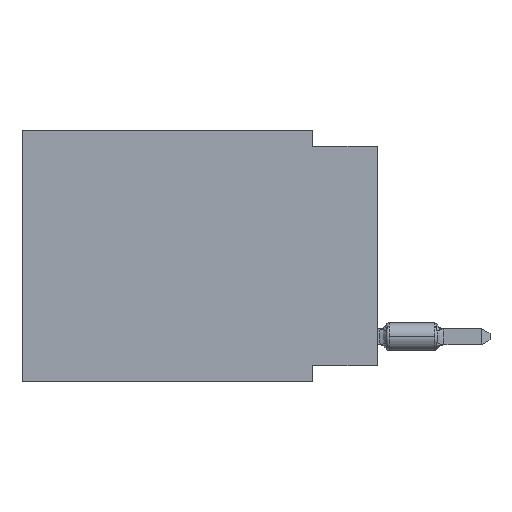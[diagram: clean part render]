
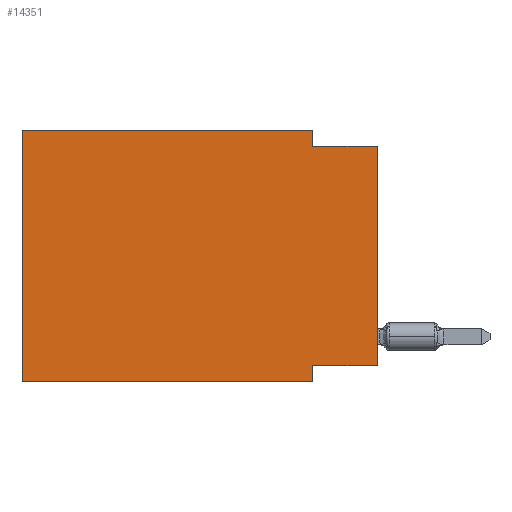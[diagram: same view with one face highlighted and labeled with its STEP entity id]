
A CAD part, left-side view. The second image highlights one B-rep face of the part: STEP entity #14351.
In plain terms, the highlighted planar face has unit normal (-1, 0, 0).
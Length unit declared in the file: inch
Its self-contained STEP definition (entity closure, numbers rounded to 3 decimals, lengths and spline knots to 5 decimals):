
#450 = DIRECTION ( 'NONE',  ( 0., 0., -1. ) ) ;
#493 = CARTESIAN_POINT ( 'NONE',  ( 0., 0.1, -0.39 ) ) ;
#547 = EDGE_CURVE ( 'NONE', #9017, #11128, #4218, .T. ) ;
#748 = DIRECTION ( 'NONE',  ( 0., 0., -1. ) ) ;
#989 = CARTESIAN_POINT ( 'NONE',  ( 0., 0.1, -0.365 ) ) ;
#1111 = CARTESIAN_POINT ( 'NONE',  ( 0., 0., -0.365 ) ) ;
#1274 = DIRECTION ( 'NONE',  ( 0., 0., -1. ) ) ;
#1516 = EDGE_CURVE ( 'NONE', #4479, #1922, #7244, .T. ) ;
#1914 = EDGE_CURVE ( 'NONE', #4148, #11128, #11303, .T. ) ;
#1922 = VERTEX_POINT ( 'NONE', #7546 ) ;
#2011 = ORIENTED_EDGE ( 'NONE', *, *, #15086, .T. ) ;
#2203 = CARTESIAN_POINT ( 'NONE',  ( 0., 0., -0.025 ) ) ;
#2472 = DIRECTION ( 'NONE',  ( 0., 1., 0. ) ) ;
#2761 = ORIENTED_EDGE ( 'NONE', *, *, #13108, .F. ) ;
#2795 = CARTESIAN_POINT ( 'NONE',  ( 0., 0., -0.365 ) ) ;
#2807 = CARTESIAN_POINT ( 'NONE',  ( 0., 0.1, 0. ) ) ;
#3110 = CARTESIAN_POINT ( 'NONE',  ( 0., 0.55, -0.39 ) ) ;
#3275 = LINE ( 'NONE', #16688, #9302 ) ;
#3716 = LINE ( 'NONE', #4912, #11057 ) ;
#4130 = VECTOR ( 'NONE', #748, 39.37008 ) ;
#4148 = VERTEX_POINT ( 'NONE', #2795 ) ;
#4209 = CARTESIAN_POINT ( 'NONE',  ( 0., 0.1, 0. ) ) ;
#4218 = LINE ( 'NONE', #9438, #11420 ) ;
#4401 = CARTESIAN_POINT ( 'NONE',  ( 0., 0.1, -0.025 ) ) ;
#4479 = VERTEX_POINT ( 'NONE', #989 ) ;
#4912 = CARTESIAN_POINT ( 'NONE',  ( 0., 0.55, -0.39 ) ) ;
#5392 = AXIS2_PLACEMENT_3D ( 'NONE', #11534, #10338, #1274 ) ;
#6012 = CARTESIAN_POINT ( 'NONE',  ( 0., 0., 0. ) ) ;
#6150 = ORIENTED_EDGE ( 'NONE', *, *, #10513, .F. ) ;
#6856 = DIRECTION ( 'NONE',  ( 0., -1., 0. ) ) ;
#7154 = EDGE_CURVE ( 'NONE', #13836, #11125, #3275, .T. ) ;
#7244 = LINE ( 'NONE', #493, #4130 ) ;
#7546 = CARTESIAN_POINT ( 'NONE',  ( 0., 0.1, -0.39 ) ) ;
#8159 = DIRECTION ( 'NONE',  ( 0., -1., 0. ) ) ;
#8424 = VECTOR ( 'NONE', #450, 39.37008 ) ;
#8580 = DIRECTION ( 'NONE',  ( 0., 0., 1. ) ) ;
#8835 = EDGE_LOOP ( 'NONE', ( #12155, #10376, #6150, #11674, #10535, #2011, #12660, #2761 ) ) ;
#9017 = VERTEX_POINT ( 'NONE', #4401 ) ;
#9302 = VECTOR ( 'NONE', #8580, 39.37008 ) ;
#9438 = CARTESIAN_POINT ( 'NONE',  ( 0., 0., -0.025 ) ) ;
#9688 = VERTEX_POINT ( 'NONE', #2807 ) ;
#10018 = VECTOR ( 'NONE', #2472, 39.37008 ) ;
#10338 = DIRECTION ( 'NONE',  ( 1., 0., 0. ) ) ;
#10376 = ORIENTED_EDGE ( 'NONE', *, *, #547, .F. ) ;
#10513 = EDGE_CURVE ( 'NONE', #9688, #9017, #13530, .T. ) ;
#10535 = ORIENTED_EDGE ( 'NONE', *, *, #7154, .F. ) ;
#10608 = LINE ( 'NONE', #13252, #14304 ) ;
#11057 = VECTOR ( 'NONE', #16623, 39.37008 ) ;
#11125 = VERTEX_POINT ( 'NONE', #11599 ) ;
#11128 = VERTEX_POINT ( 'NONE', #2203 ) ;
#11303 = LINE ( 'NONE', #6012, #16416 ) ;
#11420 = VECTOR ( 'NONE', #8159, 39.37008 ) ;
#11534 = CARTESIAN_POINT ( 'NONE',  ( 0., 0.55, 0. ) ) ;
#11599 = CARTESIAN_POINT ( 'NONE',  ( 0., 0.55, 0. ) ) ;
#11674 = ORIENTED_EDGE ( 'NONE', *, *, #15645, .F. ) ;
#12155 = ORIENTED_EDGE ( 'NONE', *, *, #1914, .T. ) ;
#12660 = ORIENTED_EDGE ( 'NONE', *, *, #1516, .F. ) ;
#12980 = PLANE ( 'NONE',  #5392 ) ;
#13108 = EDGE_CURVE ( 'NONE', #4148, #4479, #16830, .T. ) ;
#13252 = CARTESIAN_POINT ( 'NONE',  ( 0., 0.55, 0. ) ) ;
#13530 = LINE ( 'NONE', #4209, #8424 ) ;
#13836 = VERTEX_POINT ( 'NONE', #3110 ) ;
#14304 = VECTOR ( 'NONE', #6856, 39.37008 ) ;
#14351 = ADVANCED_FACE ( 'NONE', ( #16834 ), #12980, .F. ) ;
#15086 = EDGE_CURVE ( 'NONE', #13836, #1922, #3716, .T. ) ;
#15645 = EDGE_CURVE ( 'NONE', #11125, #9688, #10608, .T. ) ;
#16416 = VECTOR ( 'NONE', #16521, 39.37008 ) ;
#16521 = DIRECTION ( 'NONE',  ( 0., 0., 1. ) ) ;
#16623 = DIRECTION ( 'NONE',  ( 0., -1., 0. ) ) ;
#16688 = CARTESIAN_POINT ( 'NONE',  ( 0., 0.55, 0. ) ) ;
#16830 = LINE ( 'NONE', #1111, #10018 ) ;
#16834 = FACE_OUTER_BOUND ( 'NONE', #8835, .T. ) ;
